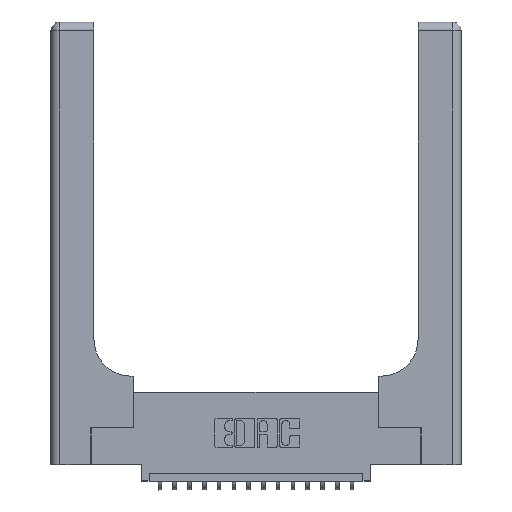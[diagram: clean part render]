
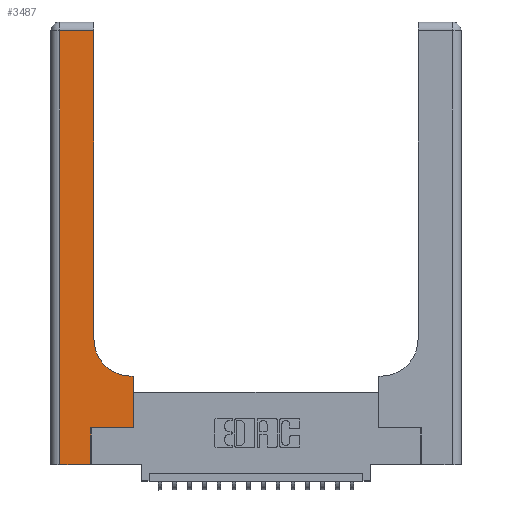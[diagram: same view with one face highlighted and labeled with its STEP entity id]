
A CAD part, top view. The second image highlights one B-rep face of the part: STEP entity #3487.
In plain terms, the highlighted planar face has unit normal (0, 0, 1).
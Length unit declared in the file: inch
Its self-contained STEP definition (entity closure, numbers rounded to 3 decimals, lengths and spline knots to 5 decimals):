
#427 = EDGE_CURVE ( 'NONE', #10564, #7013, #11454, .T. ) ;
#674 = VECTOR ( 'NONE', #11586, 39.37008 ) ;
#990 = CARTESIAN_POINT ( 'NONE',  ( 0., 3., 0.37 ) ) ;
#1563 = ORIENTED_EDGE ( 'NONE', *, *, #7988, .T. ) ;
#1616 = LINE ( 'NONE', #15281, #4447 ) ;
#1740 = VERTEX_POINT ( 'NONE', #18557 ) ;
#1852 = CARTESIAN_POINT ( 'NONE',  ( 0.269, 0., 0.37 ) ) ;
#2028 = DIRECTION ( 'NONE',  ( -1., 0., 0. ) ) ;
#2396 = VECTOR ( 'NONE', #16519, 39.37008 ) ;
#3242 = EDGE_LOOP ( 'NONE', ( #9568, #18715, #10255, #19187, #16725, #7737, #1563, #12718, #15846 ) ) ;
#3487 = ADVANCED_FACE ( 'NONE', ( #15889 ), #9872, .F. ) ;
#3939 = CARTESIAN_POINT ( 'NONE',  ( 0., 2.94, 0.37 ) ) ;
#4140 = EDGE_CURVE ( 'NONE', #1740, #10564, #8218, .T. ) ;
#4429 = AXIS2_PLACEMENT_3D ( 'NONE', #14466, #5330, #19205 ) ;
#4447 = VECTOR ( 'NONE', #4934, 39.37008 ) ;
#4705 = LINE ( 'NONE', #14912, #674 ) ;
#4934 = DIRECTION ( 'NONE',  ( 1., 0., 0. ) ) ;
#5119 = VECTOR ( 'NONE', #13507, 39.37008 ) ;
#5149 = CARTESIAN_POINT ( 'NONE',  ( 0.269, 0.25, 0.37 ) ) ;
#5330 = DIRECTION ( 'NONE',  ( 0., 0., -1. ) ) ;
#6649 = VECTOR ( 'NONE', #6929, 39.37008 ) ;
#6929 = DIRECTION ( 'NONE',  ( 0., 1., 0. ) ) ;
#7013 = VERTEX_POINT ( 'NONE', #1852 ) ;
#7499 = CARTESIAN_POINT ( 'NONE',  ( 0.5585, 0.25, 0.37 ) ) ;
#7509 = EDGE_CURVE ( 'NONE', #19119, #7886, #11879, .T. ) ;
#7737 = ORIENTED_EDGE ( 'NONE', *, *, #13347, .T. ) ;
#7886 = VERTEX_POINT ( 'NONE', #10056 ) ;
#7988 = EDGE_CURVE ( 'NONE', #16996, #10376, #12801, .T. ) ;
#8218 = LINE ( 'NONE', #8925, #5119 ) ;
#8925 = CARTESIAN_POINT ( 'NONE',  ( 0.06, 3., 0.37 ) ) ;
#9568 = ORIENTED_EDGE ( 'NONE', *, *, #14327, .T. ) ;
#9872 = PLANE ( 'NONE',  #18404 ) ;
#10056 = CARTESIAN_POINT ( 'NONE',  ( 0.2915, 0.85, 0.37 ) ) ;
#10255 = ORIENTED_EDGE ( 'NONE', *, *, #4140, .T. ) ;
#10297 = CARTESIAN_POINT ( 'NONE',  ( 0.5415, 0.6, 0.37 ) ) ;
#10376 = VERTEX_POINT ( 'NONE', #19653 ) ;
#10564 = VERTEX_POINT ( 'NONE', #12753 ) ;
#10794 = EDGE_CURVE ( 'NONE', #7013, #14019, #18640, .T. ) ;
#11454 = LINE ( 'NONE', #18197, #2396 ) ;
#11586 = DIRECTION ( 'NONE',  ( -1., 0., 0. ) ) ;
#11879 = CIRCLE ( 'NONE', #4429, 0.25 ) ;
#12192 = EDGE_CURVE ( 'NONE', #14824, #1740, #19057, .T. ) ;
#12697 = CARTESIAN_POINT ( 'NONE',  ( 0.2915, 3., 0.37 ) ) ;
#12718 = ORIENTED_EDGE ( 'NONE', *, *, #12928, .T. ) ;
#12753 = CARTESIAN_POINT ( 'NONE',  ( 0.06, 0., 0.37 ) ) ;
#12801 = LINE ( 'NONE', #19127, #6649 ) ;
#12928 = EDGE_CURVE ( 'NONE', #10376, #19119, #4705, .T. ) ;
#13347 = EDGE_CURVE ( 'NONE', #14019, #16996, #1616, .T. ) ;
#13507 = DIRECTION ( 'NONE',  ( 0., -1., 0. ) ) ;
#14019 = VERTEX_POINT ( 'NONE', #5149 ) ;
#14278 = VECTOR ( 'NONE', #16187, 39.37008 ) ;
#14327 = EDGE_CURVE ( 'NONE', #7886, #14824, #17552, .T. ) ;
#14341 = VECTOR ( 'NONE', #18031, 39.37008 ) ;
#14466 = CARTESIAN_POINT ( 'NONE',  ( 0.5415, 0.85, 0.37 ) ) ;
#14824 = VERTEX_POINT ( 'NONE', #18915 ) ;
#14912 = CARTESIAN_POINT ( 'NONE',  ( 0.2915, 0.6, 0.37 ) ) ;
#15281 = CARTESIAN_POINT ( 'NONE',  ( 0.269, 0.25, 0.37 ) ) ;
#15802 = DIRECTION ( 'NONE',  ( 0., 1., 0. ) ) ;
#15846 = ORIENTED_EDGE ( 'NONE', *, *, #7509, .T. ) ;
#15889 = FACE_OUTER_BOUND ( 'NONE', #3242, .T. ) ;
#16187 = DIRECTION ( 'NONE',  ( -1., 0., 0. ) ) ;
#16519 = DIRECTION ( 'NONE',  ( 1., 0., 0. ) ) ;
#16725 = ORIENTED_EDGE ( 'NONE', *, *, #10794, .T. ) ;
#16996 = VERTEX_POINT ( 'NONE', #7499 ) ;
#17552 = LINE ( 'NONE', #12697, #19682 ) ;
#17976 = DIRECTION ( 'NONE',  ( 0., 0., -1. ) ) ;
#18031 = DIRECTION ( 'NONE',  ( 0., 1., 0. ) ) ;
#18197 = CARTESIAN_POINT ( 'NONE',  ( 0., 0., 0.37 ) ) ;
#18404 = AXIS2_PLACEMENT_3D ( 'NONE', #990, #17976, #2028 ) ;
#18557 = CARTESIAN_POINT ( 'NONE',  ( 0.06, 2.94, 0.37 ) ) ;
#18640 = LINE ( 'NONE', #19624, #14341 ) ;
#18715 = ORIENTED_EDGE ( 'NONE', *, *, #12192, .T. ) ;
#18915 = CARTESIAN_POINT ( 'NONE',  ( 0.2915, 2.94, 0.37 ) ) ;
#19057 = LINE ( 'NONE', #3939, #14278 ) ;
#19119 = VERTEX_POINT ( 'NONE', #10297 ) ;
#19127 = CARTESIAN_POINT ( 'NONE',  ( 0.5585, 0.25, 0.37 ) ) ;
#19187 = ORIENTED_EDGE ( 'NONE', *, *, #427, .T. ) ;
#19205 = DIRECTION ( 'NONE',  ( 1., 0., 0. ) ) ;
#19624 = CARTESIAN_POINT ( 'NONE',  ( 0.269, 0., 0.37 ) ) ;
#19653 = CARTESIAN_POINT ( 'NONE',  ( 0.5585, 0.6, 0.37 ) ) ;
#19682 = VECTOR ( 'NONE', #15802, 39.37008 ) ;
